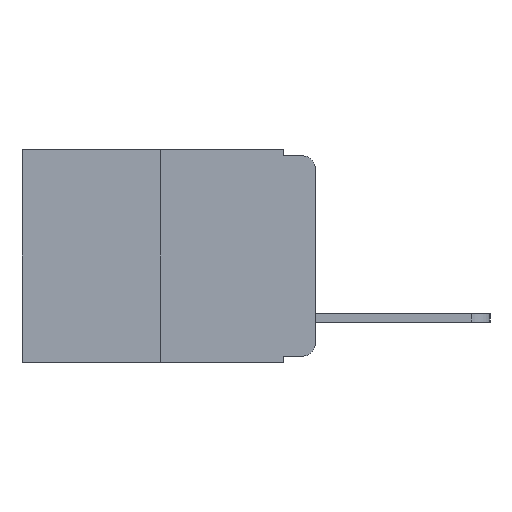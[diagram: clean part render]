
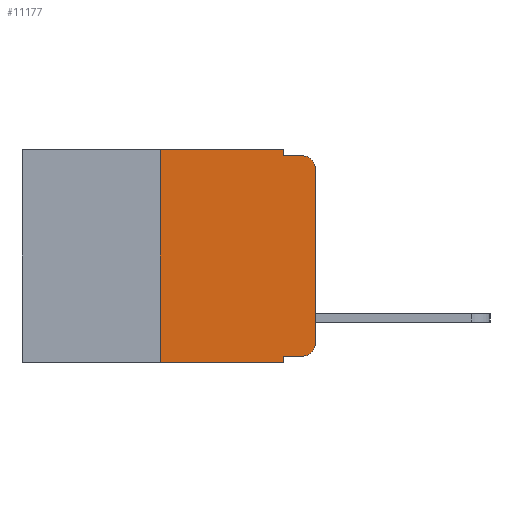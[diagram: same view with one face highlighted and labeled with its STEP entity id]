
A CAD part, left-side view. The second image highlights one B-rep face of the part: STEP entity #11177.
In plain terms, the highlighted planar face has unit normal (-1, 0, 0).
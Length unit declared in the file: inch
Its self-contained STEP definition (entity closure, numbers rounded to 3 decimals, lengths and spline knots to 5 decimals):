
#58 = EDGE_CURVE ( 'NONE', #18908, #9918, #8657, .T. ) ;
#412 = ORIENTED_EDGE ( 'NONE', *, *, #9364, .F. ) ;
#618 = EDGE_CURVE ( 'NONE', #18512, #9918, #10885, .T. ) ;
#1476 = CARTESIAN_POINT ( 'NONE',  ( 0., 0.02, -0.01 ) ) ;
#2018 = DIRECTION ( 'NONE',  ( -1., 0., 0. ) ) ;
#2030 = EDGE_CURVE ( 'NONE', #21563, #8987, #19389, .T. ) ;
#2050 = DIRECTION ( 'NONE',  ( 0., 0., -1. ) ) ;
#2590 = DIRECTION ( 'NONE',  ( 0., 0., -1. ) ) ;
#3002 = LINE ( 'NONE', #6382, #12020 ) ;
#3366 = DIRECTION ( 'NONE',  ( -1., 0., 0. ) ) ;
#3425 = ORIENTED_EDGE ( 'NONE', *, *, #13968, .F. ) ;
#3484 = LINE ( 'NONE', #6066, #7265 ) ;
#3584 = DIRECTION ( 'NONE',  ( 0., -1., 0. ) ) ;
#4016 = EDGE_CURVE ( 'NONE', #21753, #18512, #18041, .T. ) ;
#4020 = ORIENTED_EDGE ( 'NONE', *, *, #16294, .T. ) ;
#4265 = LINE ( 'NONE', #16919, #21385 ) ;
#4530 = CARTESIAN_POINT ( 'NONE',  ( 0., 0.02, -0.03 ) ) ;
#4974 = CARTESIAN_POINT ( 'NONE',  ( 0., 0.473, -0.343 ) ) ;
#4977 = DIRECTION ( 'NONE',  ( 1., 0., 0. ) ) ;
#5052 = VERTEX_POINT ( 'NONE', #16849 ) ;
#5403 = DIRECTION ( 'NONE',  ( 0., 0., 1. ) ) ;
#5504 = ORIENTED_EDGE ( 'NONE', *, *, #18006, .F. ) ;
#5593 = DIRECTION ( 'NONE',  ( 0., -1., 0. ) ) ;
#5861 = VERTEX_POINT ( 'NONE', #19176 ) ;
#6066 = CARTESIAN_POINT ( 'NONE',  ( 0., 0.051, 0. ) ) ;
#6287 = AXIS2_PLACEMENT_3D ( 'NONE', #14022, #3366, #15795 ) ;
#6382 = CARTESIAN_POINT ( 'NONE',  ( 0., 0.051, 0. ) ) ;
#7265 = VECTOR ( 'NONE', #19631, 39.37008 ) ;
#7594 = CARTESIAN_POINT ( 'NONE',  ( 0., 0.051, -0.333 ) ) ;
#8365 = CARTESIAN_POINT ( 'NONE',  ( 0., 0.051, -0.01 ) ) ;
#8657 = LINE ( 'NONE', #22312, #12218 ) ;
#8880 = ORIENTED_EDGE ( 'NONE', *, *, #20494, .T. ) ;
#8987 = VERTEX_POINT ( 'NONE', #21085 ) ;
#9022 = CARTESIAN_POINT ( 'NONE',  ( 0., 0.25, 0. ) ) ;
#9057 = CARTESIAN_POINT ( 'NONE',  ( 0., 0.473, 0. ) ) ;
#9364 = EDGE_CURVE ( 'NONE', #5052, #18908, #3484, .T. ) ;
#9918 = VERTEX_POINT ( 'NONE', #1476 ) ;
#10127 = DIRECTION ( 'NONE',  ( 0., -1., 0. ) ) ;
#10885 = CIRCLE ( 'NONE', #20396, 0.02 ) ;
#11177 = ADVANCED_FACE ( 'NONE', ( #21674 ), #13806, .F. ) ;
#11257 = CIRCLE ( 'NONE', #6287, 0.02 ) ;
#11703 = EDGE_CURVE ( 'NONE', #21563, #21723, #12378, .T. ) ;
#12020 = VECTOR ( 'NONE', #2590, 39.37008 ) ;
#12075 = DIRECTION ( 'NONE',  ( 0., 0., 1. ) ) ;
#12214 = CARTESIAN_POINT ( 'NONE',  ( 0., 0.25, -0.343 ) ) ;
#12218 = VECTOR ( 'NONE', #5593, 39.37008 ) ;
#12378 = LINE ( 'NONE', #20247, #20596 ) ;
#13127 = DIRECTION ( 'NONE',  ( 0., -1., 0. ) ) ;
#13158 = VERTEX_POINT ( 'NONE', #7594 ) ;
#13213 = ORIENTED_EDGE ( 'NONE', *, *, #4016, .T. ) ;
#13764 = ORIENTED_EDGE ( 'NONE', *, *, #618, .T. ) ;
#13806 = PLANE ( 'NONE',  #15672 ) ;
#13968 = EDGE_CURVE ( 'NONE', #13158, #8987, #3002, .T. ) ;
#14022 = CARTESIAN_POINT ( 'NONE',  ( 0., 0.02, -0.313 ) ) ;
#14198 = CARTESIAN_POINT ( 'NONE',  ( 0., 0., -0.313 ) ) ;
#14546 = VECTOR ( 'NONE', #13127, 39.37008 ) ;
#15391 = ORIENTED_EDGE ( 'NONE', *, *, #11703, .F. ) ;
#15558 = CARTESIAN_POINT ( 'NONE',  ( 0., 0.473, 0. ) ) ;
#15672 = AXIS2_PLACEMENT_3D ( 'NONE', #15558, #4977, #17202 ) ;
#15795 = DIRECTION ( 'NONE',  ( 0., 0., -1. ) ) ;
#16294 = EDGE_CURVE ( 'NONE', #13158, #5861, #4265, .T. ) ;
#16621 = VECTOR ( 'NONE', #3584, 39.37008 ) ;
#16849 = CARTESIAN_POINT ( 'NONE',  ( 0., 0.051, 0. ) ) ;
#16919 = CARTESIAN_POINT ( 'NONE',  ( 0., 0.051, -0.333 ) ) ;
#17033 = EDGE_LOOP ( 'NONE', ( #13213, #13764, #18174, #412, #5504, #15391, #19628, #3425, #4020, #8880 ) ) ;
#17202 = DIRECTION ( 'NONE',  ( 0., 0., -1. ) ) ;
#17557 = VECTOR ( 'NONE', #5403, 39.37008 ) ;
#18006 = EDGE_CURVE ( 'NONE', #21723, #5052, #20805, .T. ) ;
#18041 = LINE ( 'NONE', #20613, #17557 ) ;
#18174 = ORIENTED_EDGE ( 'NONE', *, *, #58, .F. ) ;
#18512 = VERTEX_POINT ( 'NONE', #21512 ) ;
#18908 = VERTEX_POINT ( 'NONE', #8365 ) ;
#19176 = CARTESIAN_POINT ( 'NONE',  ( 0., 0.02, -0.333 ) ) ;
#19389 = LINE ( 'NONE', #4974, #14546 ) ;
#19628 = ORIENTED_EDGE ( 'NONE', *, *, #2030, .T. ) ;
#19631 = DIRECTION ( 'NONE',  ( 0., 0., -1. ) ) ;
#20247 = CARTESIAN_POINT ( 'NONE',  ( 0., 0.25, 0. ) ) ;
#20396 = AXIS2_PLACEMENT_3D ( 'NONE', #4530, #2018, #2050 ) ;
#20494 = EDGE_CURVE ( 'NONE', #5861, #21753, #11257, .T. ) ;
#20596 = VECTOR ( 'NONE', #12075, 39.37008 ) ;
#20613 = CARTESIAN_POINT ( 'NONE',  ( 0., 0., 0. ) ) ;
#20805 = LINE ( 'NONE', #9057, #16621 ) ;
#21085 = CARTESIAN_POINT ( 'NONE',  ( 0., 0.051, -0.343 ) ) ;
#21385 = VECTOR ( 'NONE', #10127, 39.37008 ) ;
#21512 = CARTESIAN_POINT ( 'NONE',  ( 0., 0., -0.03 ) ) ;
#21563 = VERTEX_POINT ( 'NONE', #12214 ) ;
#21674 = FACE_OUTER_BOUND ( 'NONE', #17033, .T. ) ;
#21723 = VERTEX_POINT ( 'NONE', #9022 ) ;
#21753 = VERTEX_POINT ( 'NONE', #14198 ) ;
#22312 = CARTESIAN_POINT ( 'NONE',  ( 0., 0.051, -0.01 ) ) ;
